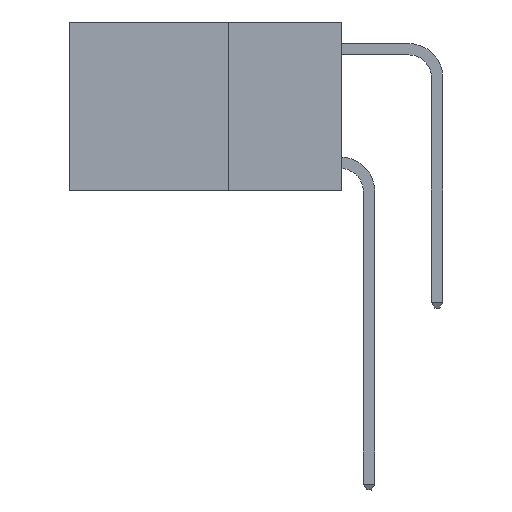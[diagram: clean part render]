
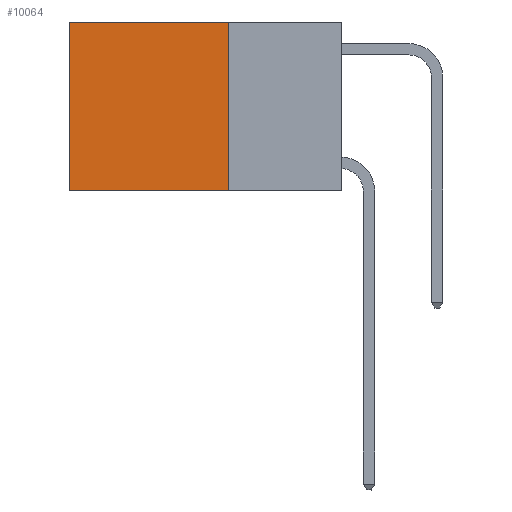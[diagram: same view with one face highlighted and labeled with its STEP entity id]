
A CAD part, left-side view. The second image highlights one B-rep face of the part: STEP entity #10064.
In plain terms, the highlighted planar face has unit normal (-1, 0, 0).
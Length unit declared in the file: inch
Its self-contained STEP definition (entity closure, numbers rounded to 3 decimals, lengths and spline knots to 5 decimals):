
#189 = EDGE_CURVE ( 'NONE', #2277, #10454, #5357, .T. ) ;
#287 = DIRECTION ( 'NONE',  ( 0., 1., 0. ) ) ;
#376 = DIRECTION ( 'NONE',  ( 0., 0., -1. ) ) ;
#388 = VECTOR ( 'NONE', #376, 39.37008 ) ;
#936 = DIRECTION ( 'NONE',  ( 1., 0., 0. ) ) ;
#1845 = DIRECTION ( 'NONE',  ( 0., 1., 0. ) ) ;
#1984 = CARTESIAN_POINT ( 'NONE',  ( 0.2625, 0.25, 0. ) ) ;
#2277 = VERTEX_POINT ( 'NONE', #10188 ) ;
#2516 = ORIENTED_EDGE ( 'NONE', *, *, #10557, .T. ) ;
#2609 = ORIENTED_EDGE ( 'NONE', *, *, #8466, .T. ) ;
#4284 = LINE ( 'NONE', #10615, #388 ) ;
#4411 = VECTOR ( 'NONE', #287, 39.37008 ) ;
#4897 = ORIENTED_EDGE ( 'NONE', *, *, #7457, .F. ) ;
#5049 = VERTEX_POINT ( 'NONE', #5431 ) ;
#5357 = LINE ( 'NONE', #10660, #4411 ) ;
#5431 = CARTESIAN_POINT ( 'NONE',  ( 0.2625, 0.6, 0. ) ) ;
#5733 = EDGE_LOOP ( 'NONE', ( #2609, #8531, #4897, #2516 ) ) ;
#5820 = CARTESIAN_POINT ( 'NONE',  ( 0.2625, 0.6, 0. ) ) ;
#6054 = PLANE ( 'NONE',  #7155 ) ;
#6463 = LINE ( 'NONE', #1984, #10320 ) ;
#6881 = CARTESIAN_POINT ( 'NONE',  ( 0.2625, 0.25, 0. ) ) ;
#6882 = VERTEX_POINT ( 'NONE', #10376 ) ;
#6931 = DIRECTION ( 'NONE',  ( 0., 0., -1. ) ) ;
#7155 = AXIS2_PLACEMENT_3D ( 'NONE', #6881, #936, #6931 ) ;
#7457 = EDGE_CURVE ( 'NONE', #6882, #2277, #4284, .T. ) ;
#7638 = CARTESIAN_POINT ( 'NONE',  ( 0.2625, 0.6, -0.37 ) ) ;
#8044 = VECTOR ( 'NONE', #9224, 39.37008 ) ;
#8466 = EDGE_CURVE ( 'NONE', #5049, #10454, #10342, .T. ) ;
#8531 = ORIENTED_EDGE ( 'NONE', *, *, #189, .F. ) ;
#8717 = FACE_OUTER_BOUND ( 'NONE', #5733, .T. ) ;
#9224 = DIRECTION ( 'NONE',  ( 0., 0., -1. ) ) ;
#10064 = ADVANCED_FACE ( 'NONE', ( #8717 ), #6054, .F. ) ;
#10188 = CARTESIAN_POINT ( 'NONE',  ( 0.2625, 0.25, -0.37 ) ) ;
#10320 = VECTOR ( 'NONE', #1845, 39.37008 ) ;
#10342 = LINE ( 'NONE', #5820, #8044 ) ;
#10376 = CARTESIAN_POINT ( 'NONE',  ( 0.2625, 0.25, 0. ) ) ;
#10454 = VERTEX_POINT ( 'NONE', #7638 ) ;
#10557 = EDGE_CURVE ( 'NONE', #6882, #5049, #6463, .T. ) ;
#10615 = CARTESIAN_POINT ( 'NONE',  ( 0.2625, 0.25, 0. ) ) ;
#10660 = CARTESIAN_POINT ( 'NONE',  ( 0.2625, 0.25, -0.37 ) ) ;
